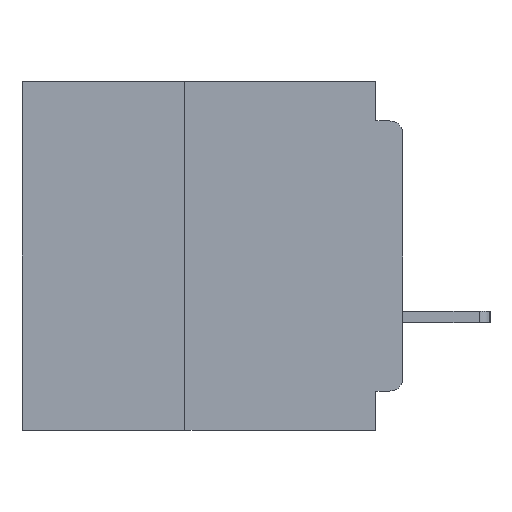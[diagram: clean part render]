
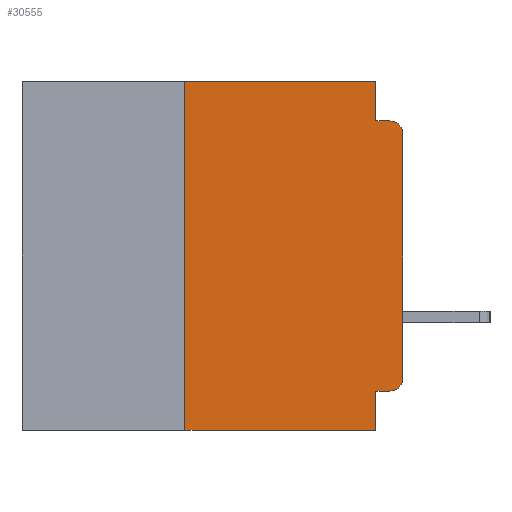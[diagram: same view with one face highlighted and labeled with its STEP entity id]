
A CAD part, left-side view. The second image highlights one B-rep face of the part: STEP entity #30555.
In plain terms, the highlighted planar face has unit normal (-1, 0, 0).
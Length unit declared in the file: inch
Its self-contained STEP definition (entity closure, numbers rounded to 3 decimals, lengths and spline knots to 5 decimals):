
#11 = LINE ( 'NONE', #35948, #30361 ) ;
#340 = DIRECTION ( 'NONE',  ( -1., 0., 0. ) ) ;
#449 = CARTESIAN_POINT ( 'NONE',  ( 0., 0.031, -0.355 ) ) ;
#1236 = VECTOR ( 'NONE', #4324, 39.37008 ) ;
#1977 = EDGE_CURVE ( 'NONE', #5724, #17381, #11, .T. ) ;
#2540 = VERTEX_POINT ( 'NONE', #9555 ) ;
#2575 = PLANE ( 'NONE',  #19154 ) ;
#2774 = CARTESIAN_POINT ( 'NONE',  ( 0., 0.437, -0.4 ) ) ;
#3730 = VERTEX_POINT ( 'NONE', #5446 ) ;
#3734 = EDGE_CURVE ( 'NONE', #5314, #3730, #16784, .T. ) ;
#3860 = CARTESIAN_POINT ( 'NONE',  ( 0., 0., -0.045 ) ) ;
#3993 = CIRCLE ( 'NONE', #15161, 0.015 ) ;
#4324 = DIRECTION ( 'NONE',  ( 0., 0., -1. ) ) ;
#4500 = CARTESIAN_POINT ( 'NONE',  ( 0., 0.031, 0. ) ) ;
#4898 = ORIENTED_EDGE ( 'NONE', *, *, #14044, .F. ) ;
#5306 = DIRECTION ( 'NONE',  ( 0., 0., -1. ) ) ;
#5314 = VERTEX_POINT ( 'NONE', #21052 ) ;
#5405 = EDGE_LOOP ( 'NONE', ( #15778, #33299, #4898, #20307, #32841, #7214, #24527, #19894, #35612, #17237 ) ) ;
#5446 = CARTESIAN_POINT ( 'NONE',  ( 0., 0.031, -0.045 ) ) ;
#5724 = VERTEX_POINT ( 'NONE', #16940 ) ;
#6315 = VECTOR ( 'NONE', #16421, 39.37008 ) ;
#6317 = VECTOR ( 'NONE', #37820, 39.37008 ) ;
#6820 = CARTESIAN_POINT ( 'NONE',  ( 0., 0.25, -0.4 ) ) ;
#6927 = DIRECTION ( 'NONE',  ( -1., 0., 0. ) ) ;
#7214 = ORIENTED_EDGE ( 'NONE', *, *, #14424, .F. ) ;
#9555 = CARTESIAN_POINT ( 'NONE',  ( 0., 0.015, -0.045 ) ) ;
#10952 = DIRECTION ( 'NONE',  ( 0., -1., 0. ) ) ;
#11381 = DIRECTION ( 'NONE',  ( 0., 0., -1. ) ) ;
#11416 = LINE ( 'NONE', #25702, #26085 ) ;
#11781 = VECTOR ( 'NONE', #10952, 39.37008 ) ;
#11840 = EDGE_CURVE ( 'NONE', #17381, #18511, #11416, .T. ) ;
#12988 = CARTESIAN_POINT ( 'NONE',  ( 0., 0., 0. ) ) ;
#13564 = CARTESIAN_POINT ( 'NONE',  ( 0., 0., -0.34 ) ) ;
#13645 = VERTEX_POINT ( 'NONE', #13564 ) ;
#13854 = AXIS2_PLACEMENT_3D ( 'NONE', #24360, #6927, #27378 ) ;
#13998 = LINE ( 'NONE', #12988, #6315 ) ;
#13999 = LINE ( 'NONE', #2774, #6317 ) ;
#14044 = EDGE_CURVE ( 'NONE', #3730, #2540, #21267, .T. ) ;
#14424 = EDGE_CURVE ( 'NONE', #32679, #37431, #24551, .T. ) ;
#14479 = EDGE_CURVE ( 'NONE', #32679, #18511, #13999, .T. ) ;
#14812 = FACE_OUTER_BOUND ( 'NONE', #5405, .T. ) ;
#15161 = AXIS2_PLACEMENT_3D ( 'NONE', #17850, #340, #20787 ) ;
#15778 = ORIENTED_EDGE ( 'NONE', *, *, #15804, .T. ) ;
#15804 = EDGE_CURVE ( 'NONE', #13645, #27104, #13998, .T. ) ;
#16421 = DIRECTION ( 'NONE',  ( 0., 0., 1. ) ) ;
#16784 = LINE ( 'NONE', #4500, #1236 ) ;
#16940 = CARTESIAN_POINT ( 'NONE',  ( 0., 0.015, -0.355 ) ) ;
#17049 = CARTESIAN_POINT ( 'NONE',  ( 0., 0.25, -0.4 ) ) ;
#17237 = ORIENTED_EDGE ( 'NONE', *, *, #19758, .T. ) ;
#17381 = VERTEX_POINT ( 'NONE', #449 ) ;
#17850 = CARTESIAN_POINT ( 'NONE',  ( 0., 0.015, -0.06 ) ) ;
#18511 = VERTEX_POINT ( 'NONE', #24323 ) ;
#19154 = AXIS2_PLACEMENT_3D ( 'NONE', #25974, #28998, #11381 ) ;
#19523 = LINE ( 'NONE', #34438, #11781 ) ;
#19758 = EDGE_CURVE ( 'NONE', #5724, #13645, #26105, .T. ) ;
#19894 = ORIENTED_EDGE ( 'NONE', *, *, #11840, .F. ) ;
#20121 = CARTESIAN_POINT ( 'NONE',  ( 0., 0.25, 0. ) ) ;
#20307 = ORIENTED_EDGE ( 'NONE', *, *, #3734, .F. ) ;
#20787 = DIRECTION ( 'NONE',  ( 0., 0., -1. ) ) ;
#21052 = CARTESIAN_POINT ( 'NONE',  ( 0., 0.031, 0. ) ) ;
#21267 = LINE ( 'NONE', #3860, #28256 ) ;
#23459 = DIRECTION ( 'NONE',  ( 0., 1., 0. ) ) ;
#23611 = VECTOR ( 'NONE', #25787, 39.37008 ) ;
#24323 = CARTESIAN_POINT ( 'NONE',  ( 0., 0.031, -0.4 ) ) ;
#24360 = CARTESIAN_POINT ( 'NONE',  ( 0., 0.015, -0.34 ) ) ;
#24527 = ORIENTED_EDGE ( 'NONE', *, *, #14479, .T. ) ;
#24551 = LINE ( 'NONE', #17049, #23611 ) ;
#25270 = EDGE_CURVE ( 'NONE', #37431, #5314, #19523, .T. ) ;
#25702 = CARTESIAN_POINT ( 'NONE',  ( 0., 0.031, -0.4 ) ) ;
#25787 = DIRECTION ( 'NONE',  ( 0., 0., 1. ) ) ;
#25974 = CARTESIAN_POINT ( 'NONE',  ( 0., 0.437, 0. ) ) ;
#26085 = VECTOR ( 'NONE', #5306, 39.37008 ) ;
#26105 = CIRCLE ( 'NONE', #13854, 0.015 ) ;
#26165 = EDGE_CURVE ( 'NONE', #27104, #2540, #3993, .T. ) ;
#26564 = CARTESIAN_POINT ( 'NONE',  ( 0., 0., -0.06 ) ) ;
#27104 = VERTEX_POINT ( 'NONE', #26564 ) ;
#27378 = DIRECTION ( 'NONE',  ( 0., 0., -1. ) ) ;
#28256 = VECTOR ( 'NONE', #33086, 39.37008 ) ;
#28998 = DIRECTION ( 'NONE',  ( 1., 0., 0. ) ) ;
#30361 = VECTOR ( 'NONE', #23459, 39.37008 ) ;
#30555 = ADVANCED_FACE ( 'NONE', ( #14812 ), #2575, .F. ) ;
#32679 = VERTEX_POINT ( 'NONE', #6820 ) ;
#32841 = ORIENTED_EDGE ( 'NONE', *, *, #25270, .F. ) ;
#33086 = DIRECTION ( 'NONE',  ( 0., -1., 0. ) ) ;
#33299 = ORIENTED_EDGE ( 'NONE', *, *, #26165, .T. ) ;
#34438 = CARTESIAN_POINT ( 'NONE',  ( 0., 0.437, 0. ) ) ;
#35612 = ORIENTED_EDGE ( 'NONE', *, *, #1977, .F. ) ;
#35948 = CARTESIAN_POINT ( 'NONE',  ( 0., 0., -0.355 ) ) ;
#37431 = VERTEX_POINT ( 'NONE', #20121 ) ;
#37820 = DIRECTION ( 'NONE',  ( 0., -1., 0. ) ) ;
